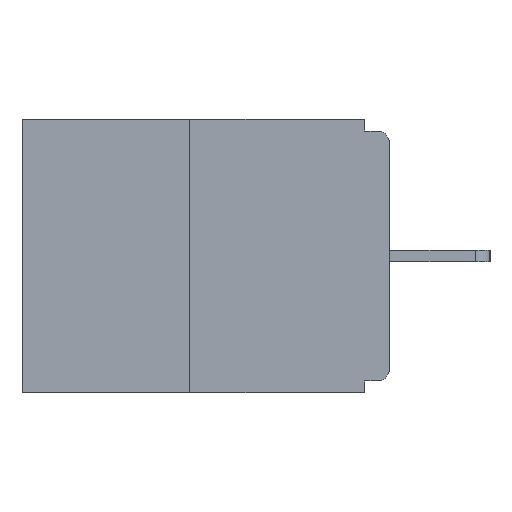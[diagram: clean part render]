
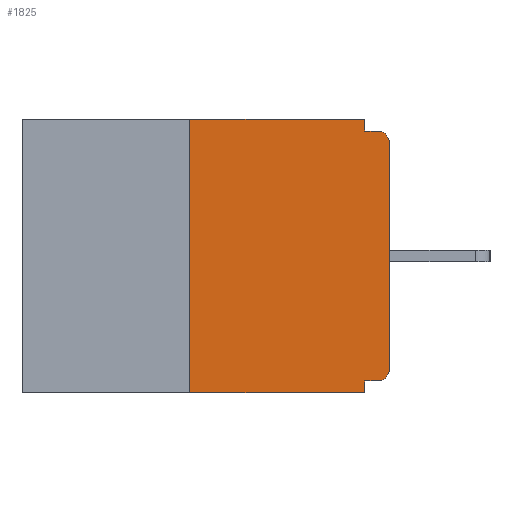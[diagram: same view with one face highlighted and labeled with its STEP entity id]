
A CAD part, left-side view. The second image highlights one B-rep face of the part: STEP entity #1825.
In plain terms, the highlighted planar face has unit normal (-1, 0, 0).
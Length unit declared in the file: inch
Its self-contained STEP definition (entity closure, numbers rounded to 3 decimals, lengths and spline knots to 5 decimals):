
#254 = DIRECTION ( 'NONE',  ( 0., 0., -1. ) ) ;
#295 = DIRECTION ( 'NONE',  ( 0., 0., 1. ) ) ;
#489 = CARTESIAN_POINT ( 'NONE',  ( 0., 0., -0.015 ) ) ;
#558 = CARTESIAN_POINT ( 'NONE',  ( 0., 0.46, 0. ) ) ;
#1082 = FACE_OUTER_BOUND ( 'NONE', #5514, .T. ) ;
#1561 = CARTESIAN_POINT ( 'NONE',  ( 0., 0.25, -0.343 ) ) ;
#1566 = VECTOR ( 'NONE', #7290, 39.37008 ) ;
#1825 = ADVANCED_FACE ( 'NONE', ( #1082 ), #7549, .F. ) ;
#2130 = ORIENTED_EDGE ( 'NONE', *, *, #12223, .F. ) ;
#2232 = ORIENTED_EDGE ( 'NONE', *, *, #8100, .F. ) ;
#2273 = AXIS2_PLACEMENT_3D ( 'NONE', #3415, #5458, #10405 ) ;
#2561 = DIRECTION ( 'NONE',  ( 0., 0., -1. ) ) ;
#2649 = CARTESIAN_POINT ( 'NONE',  ( 0., 0., -0.313 ) ) ;
#2893 = VECTOR ( 'NONE', #295, 39.37008 ) ;
#2915 = CARTESIAN_POINT ( 'NONE',  ( 0., 0.46, -0.343 ) ) ;
#3120 = VERTEX_POINT ( 'NONE', #8986 ) ;
#3172 = ORIENTED_EDGE ( 'NONE', *, *, #9895, .F. ) ;
#3283 = CARTESIAN_POINT ( 'NONE',  ( 0., 0.031, 0. ) ) ;
#3415 = CARTESIAN_POINT ( 'NONE',  ( 0., 0.015, -0.313 ) ) ;
#3529 = DIRECTION ( 'NONE',  ( 1., 0., 0. ) ) ;
#3570 = CIRCLE ( 'NONE', #2273, 0.015 ) ;
#3702 = VERTEX_POINT ( 'NONE', #3922 ) ;
#3814 = AXIS2_PLACEMENT_3D ( 'NONE', #5572, #12594, #10516 ) ;
#3922 = CARTESIAN_POINT ( 'NONE',  ( 0., 0.031, 0. ) ) ;
#3940 = EDGE_CURVE ( 'NONE', #12642, #5970, #8274, .T. ) ;
#4391 = EDGE_CURVE ( 'NONE', #3120, #10113, #3570, .T. ) ;
#4441 = CARTESIAN_POINT ( 'NONE',  ( 0., 0.46, 0. ) ) ;
#4657 = VECTOR ( 'NONE', #7825, 39.37008 ) ;
#4769 = EDGE_CURVE ( 'NONE', #6646, #5970, #4803, .T. ) ;
#4803 = CIRCLE ( 'NONE', #3814, 0.015 ) ;
#4806 = VECTOR ( 'NONE', #10224, 39.37008 ) ;
#4844 = DIRECTION ( 'NONE',  ( 0., 0., 1. ) ) ;
#5099 = VERTEX_POINT ( 'NONE', #6119 ) ;
#5458 = DIRECTION ( 'NONE',  ( -1., 0., 0. ) ) ;
#5514 = EDGE_LOOP ( 'NONE', ( #2130, #3172, #10249, #8077, #2232, #6535, #12864, #11513, #12937, #11039 ) ) ;
#5566 = VERTEX_POINT ( 'NONE', #9174 ) ;
#5572 = CARTESIAN_POINT ( 'NONE',  ( 0., 0.015, -0.03 ) ) ;
#5762 = VECTOR ( 'NONE', #7486, 39.37008 ) ;
#5853 = LINE ( 'NONE', #12303, #2893 ) ;
#5970 = VERTEX_POINT ( 'NONE', #9422 ) ;
#5985 = LINE ( 'NONE', #2915, #10373 ) ;
#6119 = CARTESIAN_POINT ( 'NONE',  ( 0., 0.031, -0.343 ) ) ;
#6535 = ORIENTED_EDGE ( 'NONE', *, *, #4391, .T. ) ;
#6646 = VERTEX_POINT ( 'NONE', #7033 ) ;
#7033 = CARTESIAN_POINT ( 'NONE',  ( 0., 0., -0.03 ) ) ;
#7095 = VECTOR ( 'NONE', #4844, 39.37008 ) ;
#7120 = VECTOR ( 'NONE', #254, 39.37008 ) ;
#7161 = VERTEX_POINT ( 'NONE', #12131 ) ;
#7224 = LINE ( 'NONE', #4441, #1566 ) ;
#7290 = DIRECTION ( 'NONE',  ( 0., -1., 0. ) ) ;
#7316 = LINE ( 'NONE', #12808, #4657 ) ;
#7486 = DIRECTION ( 'NONE',  ( 0., -1., 0. ) ) ;
#7549 = PLANE ( 'NONE',  #8989 ) ;
#7825 = DIRECTION ( 'NONE',  ( 0., 0., -1. ) ) ;
#7904 = EDGE_CURVE ( 'NONE', #7161, #5099, #7316, .T. ) ;
#8077 = ORIENTED_EDGE ( 'NONE', *, *, #7904, .F. ) ;
#8100 = EDGE_CURVE ( 'NONE', #3120, #7161, #12983, .T. ) ;
#8274 = LINE ( 'NONE', #489, #5762 ) ;
#8818 = LINE ( 'NONE', #9925, #7095 ) ;
#8986 = CARTESIAN_POINT ( 'NONE',  ( 0., 0.015, -0.328 ) ) ;
#8989 = AXIS2_PLACEMENT_3D ( 'NONE', #558, #3529, #2561 ) ;
#9174 = CARTESIAN_POINT ( 'NONE',  ( 0., 0.25, 0. ) ) ;
#9203 = VERTEX_POINT ( 'NONE', #1561 ) ;
#9213 = CARTESIAN_POINT ( 'NONE',  ( 0., 0., -0.328 ) ) ;
#9291 = CARTESIAN_POINT ( 'NONE',  ( 0., 0.031, -0.015 ) ) ;
#9301 = LINE ( 'NONE', #3283, #7120 ) ;
#9422 = CARTESIAN_POINT ( 'NONE',  ( 0., 0.015, -0.015 ) ) ;
#9506 = EDGE_CURVE ( 'NONE', #3702, #12642, #9301, .T. ) ;
#9534 = EDGE_CURVE ( 'NONE', #10113, #6646, #5853, .T. ) ;
#9895 = EDGE_CURVE ( 'NONE', #9203, #5566, #8818, .T. ) ;
#9925 = CARTESIAN_POINT ( 'NONE',  ( 0., 0.25, 0. ) ) ;
#10113 = VERTEX_POINT ( 'NONE', #2649 ) ;
#10186 = EDGE_CURVE ( 'NONE', #9203, #5099, #5985, .T. ) ;
#10224 = DIRECTION ( 'NONE',  ( 0., 1., 0. ) ) ;
#10249 = ORIENTED_EDGE ( 'NONE', *, *, #10186, .T. ) ;
#10373 = VECTOR ( 'NONE', #13004, 39.37008 ) ;
#10405 = DIRECTION ( 'NONE',  ( 0., 0., -1. ) ) ;
#10516 = DIRECTION ( 'NONE',  ( 0., 0., -1. ) ) ;
#11039 = ORIENTED_EDGE ( 'NONE', *, *, #9506, .F. ) ;
#11513 = ORIENTED_EDGE ( 'NONE', *, *, #4769, .T. ) ;
#12131 = CARTESIAN_POINT ( 'NONE',  ( 0., 0.031, -0.328 ) ) ;
#12223 = EDGE_CURVE ( 'NONE', #5566, #3702, #7224, .T. ) ;
#12303 = CARTESIAN_POINT ( 'NONE',  ( 0., 0., 0. ) ) ;
#12594 = DIRECTION ( 'NONE',  ( -1., 0., 0. ) ) ;
#12642 = VERTEX_POINT ( 'NONE', #9291 ) ;
#12808 = CARTESIAN_POINT ( 'NONE',  ( 0., 0.031, -0.343 ) ) ;
#12864 = ORIENTED_EDGE ( 'NONE', *, *, #9534, .T. ) ;
#12937 = ORIENTED_EDGE ( 'NONE', *, *, #3940, .F. ) ;
#12983 = LINE ( 'NONE', #9213, #4806 ) ;
#13004 = DIRECTION ( 'NONE',  ( 0., -1., 0. ) ) ;
